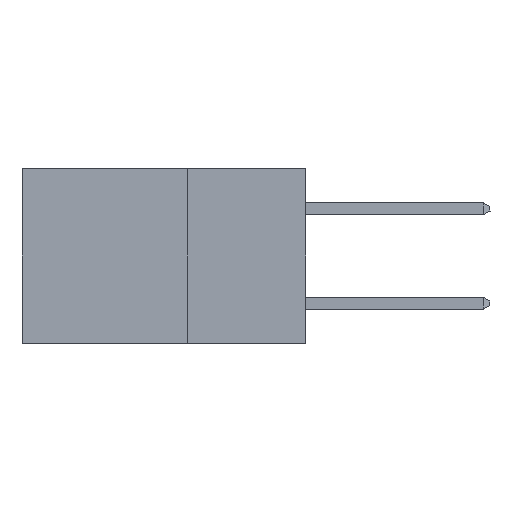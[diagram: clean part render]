
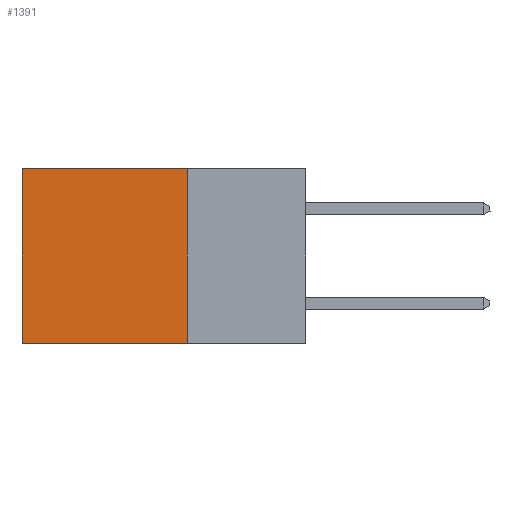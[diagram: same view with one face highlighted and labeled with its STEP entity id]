
A CAD part, left-side view. The second image highlights one B-rep face of the part: STEP entity #1391.
In plain terms, the highlighted planar face has unit normal (-1, 0, 0).
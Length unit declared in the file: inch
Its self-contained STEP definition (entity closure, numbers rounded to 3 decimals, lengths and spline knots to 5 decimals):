
#225 = VERTEX_POINT ( 'NONE', #10619 ) ;
#667 = EDGE_CURVE ( 'NONE', #7484, #18826, #6985, .T. ) ;
#1364 = CARTESIAN_POINT ( 'NONE',  ( 0.298, 0.6, 0. ) ) ;
#1391 = ADVANCED_FACE ( 'NONE', ( #9861 ), #6262, .F. ) ;
#1415 = LINE ( 'NONE', #1364, #13740 ) ;
#1542 = LINE ( 'NONE', #3389, #16648 ) ;
#1653 = EDGE_CURVE ( 'NONE', #18826, #225, #4179, .T. ) ;
#2798 = DIRECTION ( 'NONE',  ( 0., 0., -1. ) ) ;
#3389 = CARTESIAN_POINT ( 'NONE',  ( 0.298, 0.25, 0. ) ) ;
#3566 = ORIENTED_EDGE ( 'NONE', *, *, #4320, .T. ) ;
#4179 = LINE ( 'NONE', #10668, #16790 ) ;
#4320 = EDGE_CURVE ( 'NONE', #16962, #225, #1415, .T. ) ;
#4825 = CARTESIAN_POINT ( 'NONE',  ( 0.298, 0.25, -0.37 ) ) ;
#5860 = CARTESIAN_POINT ( 'NONE',  ( 0.298, 0.25, 0. ) ) ;
#6009 = CARTESIAN_POINT ( 'NONE',  ( 0.298, 0.6, 0. ) ) ;
#6262 = PLANE ( 'NONE',  #7304 ) ;
#6819 = ORIENTED_EDGE ( 'NONE', *, *, #1653, .F. ) ;
#6985 = LINE ( 'NONE', #12004, #14495 ) ;
#7304 = AXIS2_PLACEMENT_3D ( 'NONE', #16516, #7750, #17989 ) ;
#7484 = VERTEX_POINT ( 'NONE', #5860 ) ;
#7750 = DIRECTION ( 'NONE',  ( 1., 0., 0. ) ) ;
#9861 = FACE_OUTER_BOUND ( 'NONE', #18550, .T. ) ;
#10619 = CARTESIAN_POINT ( 'NONE',  ( 0.298, 0.6, -0.37 ) ) ;
#10668 = CARTESIAN_POINT ( 'NONE',  ( 0.298, 0.25, -0.37 ) ) ;
#12004 = CARTESIAN_POINT ( 'NONE',  ( 0.298, 0.25, 0. ) ) ;
#13305 = DIRECTION ( 'NONE',  ( 0., 1., 0. ) ) ;
#13534 = ORIENTED_EDGE ( 'NONE', *, *, #667, .F. ) ;
#13740 = VECTOR ( 'NONE', #2798, 39.37008 ) ;
#14495 = VECTOR ( 'NONE', #16367, 39.37008 ) ;
#16367 = DIRECTION ( 'NONE',  ( 0., 0., -1. ) ) ;
#16516 = CARTESIAN_POINT ( 'NONE',  ( 0.298, 0.25, 0. ) ) ;
#16648 = VECTOR ( 'NONE', #18138, 39.37008 ) ;
#16790 = VECTOR ( 'NONE', #13305, 39.37008 ) ;
#16962 = VERTEX_POINT ( 'NONE', #6009 ) ;
#17989 = DIRECTION ( 'NONE',  ( 0., 0., -1. ) ) ;
#18032 = ORIENTED_EDGE ( 'NONE', *, *, #18709, .T. ) ;
#18138 = DIRECTION ( 'NONE',  ( 0., 1., 0. ) ) ;
#18550 = EDGE_LOOP ( 'NONE', ( #3566, #6819, #13534, #18032 ) ) ;
#18709 = EDGE_CURVE ( 'NONE', #7484, #16962, #1542, .T. ) ;
#18826 = VERTEX_POINT ( 'NONE', #4825 ) ;
